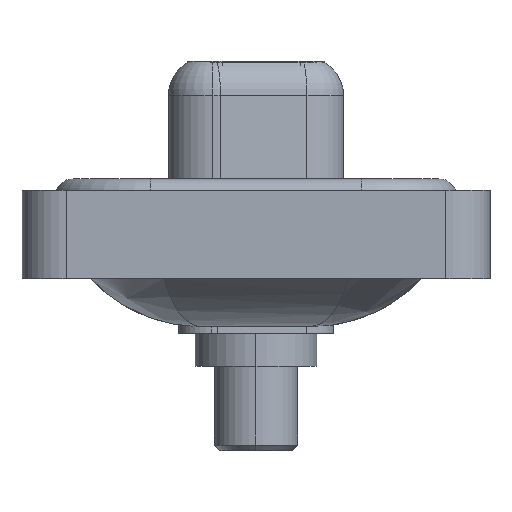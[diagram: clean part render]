
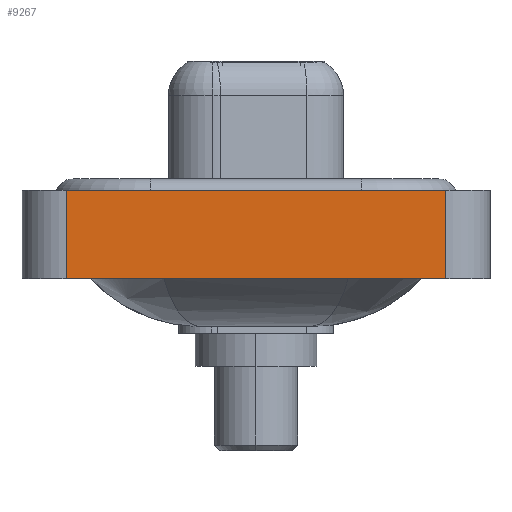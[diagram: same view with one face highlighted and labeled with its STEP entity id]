
A CAD part, left-side view. The second image highlights one B-rep face of the part: STEP entity #9267.
In plain terms, the highlighted planar face has unit normal (-1, 0, 0).
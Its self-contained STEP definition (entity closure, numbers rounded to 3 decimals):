
#301 = DIRECTION ( 'NONE',  ( 0., 0., 1. ) ) ;
#622 = LINE ( 'NONE', #14056, #14187 ) ;
#709 = EDGE_CURVE ( 'NONE', #2887, #7269, #11923, .T. ) ;
#884 = CARTESIAN_POINT ( 'NONE',  ( -7.3, -8.55, -3.6 ) ) ;
#1169 = VECTOR ( 'NONE', #301, 1000. ) ;
#2155 = CARTESIAN_POINT ( 'NONE',  ( -7.3, -8.55, -3.6 ) ) ;
#2708 = CARTESIAN_POINT ( 'NONE',  ( -7.3, -8.55, 0.4 ) ) ;
#2779 = EDGE_CURVE ( 'NONE', #7269, #14726, #622, .T. ) ;
#2887 = VERTEX_POINT ( 'NONE', #8287 ) ;
#2899 = EDGE_CURVE ( 'NONE', #8035, #14726, #8985, .T. ) ;
#4881 = ORIENTED_EDGE ( 'NONE', *, *, #2899, .F. ) ;
#5079 = LINE ( 'NONE', #9964, #1169 ) ;
#5267 = CARTESIAN_POINT ( 'NONE',  ( -7.3, -8.55, 0.4 ) ) ;
#7269 = VERTEX_POINT ( 'NONE', #2155 ) ;
#7905 = VECTOR ( 'NONE', #15671, 1000. ) ;
#8035 = VERTEX_POINT ( 'NONE', #9662 ) ;
#8287 = CARTESIAN_POINT ( 'NONE',  ( -7.3, 8.55, -3.6 ) ) ;
#8694 = DIRECTION ( 'NONE',  ( 0., -1., 0. ) ) ;
#8985 = LINE ( 'NONE', #2708, #12897 ) ;
#9267 = ADVANCED_FACE ( 'NONE', ( #9422 ), #11917, .T. ) ;
#9346 = DIRECTION ( 'NONE',  ( -1., 0., 0. ) ) ;
#9422 = FACE_OUTER_BOUND ( 'NONE', #9636, .T. ) ;
#9636 = EDGE_LOOP ( 'NONE', ( #14252, #4881, #12279, #11715 ) ) ;
#9662 = CARTESIAN_POINT ( 'NONE',  ( -7.3, 8.55, 0.4 ) ) ;
#9964 = CARTESIAN_POINT ( 'NONE',  ( -7.3, 8.55, -3.6 ) ) ;
#11433 = EDGE_CURVE ( 'NONE', #2887, #8035, #5079, .T. ) ;
#11715 = ORIENTED_EDGE ( 'NONE', *, *, #709, .T. ) ;
#11755 = CARTESIAN_POINT ( 'NONE',  ( -7.3, -8.55, -3.6 ) ) ;
#11917 = PLANE ( 'NONE',  #13879 ) ;
#11923 = LINE ( 'NONE', #884, #7905 ) ;
#12279 = ORIENTED_EDGE ( 'NONE', *, *, #11433, .F. ) ;
#12885 = DIRECTION ( 'NONE',  ( 0., 0., 1. ) ) ;
#12897 = VECTOR ( 'NONE', #8694, 1000. ) ;
#13879 = AXIS2_PLACEMENT_3D ( 'NONE', #11755, #9346, #12885 ) ;
#14056 = CARTESIAN_POINT ( 'NONE',  ( -7.3, -8.55, -3.6 ) ) ;
#14187 = VECTOR ( 'NONE', #15420, 1000. ) ;
#14252 = ORIENTED_EDGE ( 'NONE', *, *, #2779, .T. ) ;
#14726 = VERTEX_POINT ( 'NONE', #5267 ) ;
#15420 = DIRECTION ( 'NONE',  ( 0., 0., 1. ) ) ;
#15671 = DIRECTION ( 'NONE',  ( 0., -1., 0. ) ) ;
